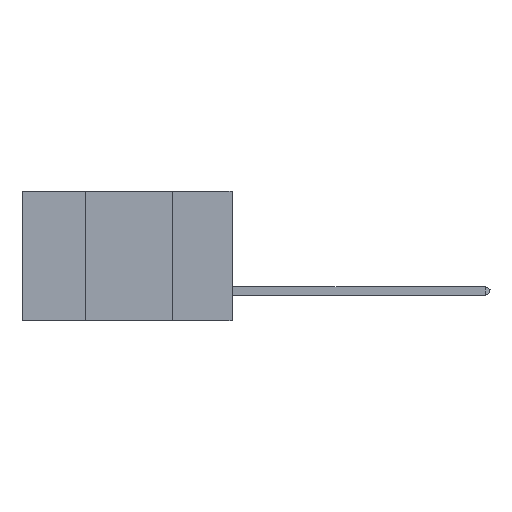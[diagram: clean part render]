
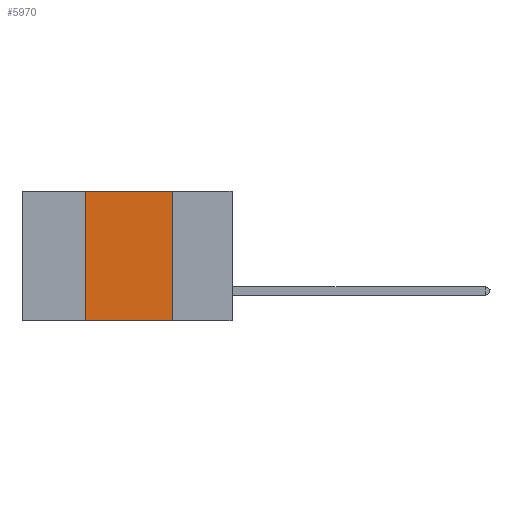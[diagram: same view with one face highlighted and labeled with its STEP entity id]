
A CAD part, left-side view. The second image highlights one B-rep face of the part: STEP entity #5970.
In plain terms, the highlighted planar face has unit normal (-1, 0, 0).
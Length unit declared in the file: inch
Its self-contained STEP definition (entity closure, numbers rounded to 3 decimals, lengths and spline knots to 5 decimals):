
#1264 = ORIENTED_EDGE ( 'NONE', *, *, #11007, .T. ) ;
#1405 = EDGE_CURVE ( 'NONE', #8235, #23438, #15972, .T. ) ;
#1550 = EDGE_LOOP ( 'NONE', ( #13749, #4734, #7951, #1264 ) ) ;
#1798 = CARTESIAN_POINT ( 'NONE',  ( 0., 0.42, 0. ) ) ;
#2268 = VERTEX_POINT ( 'NONE', #3395 ) ;
#3207 = VERTEX_POINT ( 'NONE', #23046 ) ;
#3395 = CARTESIAN_POINT ( 'NONE',  ( 0., 0.17, 0. ) ) ;
#4182 = AXIS2_PLACEMENT_3D ( 'NONE', #14152, #4365, #8973 ) ;
#4365 = DIRECTION ( 'NONE',  ( 1., 0., 0. ) ) ;
#4734 = ORIENTED_EDGE ( 'NONE', *, *, #14874, .F. ) ;
#5805 = CARTESIAN_POINT ( 'NONE',  ( 0., 0.42, 0. ) ) ;
#5970 = ADVANCED_FACE ( 'NONE', ( #10503 ), #10194, .F. ) ;
#7951 = ORIENTED_EDGE ( 'NONE', *, *, #1405, .F. ) ;
#8195 = LINE ( 'NONE', #18804, #21979 ) ;
#8235 = VERTEX_POINT ( 'NONE', #19791 ) ;
#8973 = DIRECTION ( 'NONE',  ( 0., 0., -1. ) ) ;
#9975 = VECTOR ( 'NONE', #20294, 39.37008 ) ;
#10194 = PLANE ( 'NONE',  #4182 ) ;
#10503 = FACE_OUTER_BOUND ( 'NONE', #1550, .T. ) ;
#10595 = LINE ( 'NONE', #12438, #9975 ) ;
#10912 = DIRECTION ( 'NONE',  ( 0., 0., -1. ) ) ;
#11007 = EDGE_CURVE ( 'NONE', #8235, #3207, #19632, .T. ) ;
#12438 = CARTESIAN_POINT ( 'NONE',  ( 0., 0.6, 0. ) ) ;
#12621 = EDGE_CURVE ( 'NONE', #2268, #3207, #8195, .T. ) ;
#13749 = ORIENTED_EDGE ( 'NONE', *, *, #12621, .F. ) ;
#14152 = CARTESIAN_POINT ( 'NONE',  ( 0., 0.6, 0. ) ) ;
#14874 = EDGE_CURVE ( 'NONE', #23438, #2268, #10595, .T. ) ;
#15972 = LINE ( 'NONE', #5805, #24252 ) ;
#18804 = CARTESIAN_POINT ( 'NONE',  ( 0., 0.17, 0. ) ) ;
#19632 = LINE ( 'NONE', #24867, #20574 ) ;
#19689 = DIRECTION ( 'NONE',  ( 0., 0., 1. ) ) ;
#19791 = CARTESIAN_POINT ( 'NONE',  ( 0., 0.42, -0.37 ) ) ;
#20294 = DIRECTION ( 'NONE',  ( 0., -1., 0. ) ) ;
#20574 = VECTOR ( 'NONE', #24622, 39.37008 ) ;
#21979 = VECTOR ( 'NONE', #10912, 39.37008 ) ;
#23046 = CARTESIAN_POINT ( 'NONE',  ( 0., 0.17, -0.37 ) ) ;
#23438 = VERTEX_POINT ( 'NONE', #1798 ) ;
#24252 = VECTOR ( 'NONE', #19689, 39.37008 ) ;
#24622 = DIRECTION ( 'NONE',  ( 0., -1., 0. ) ) ;
#24867 = CARTESIAN_POINT ( 'NONE',  ( 0., 0.6, -0.37 ) ) ;
